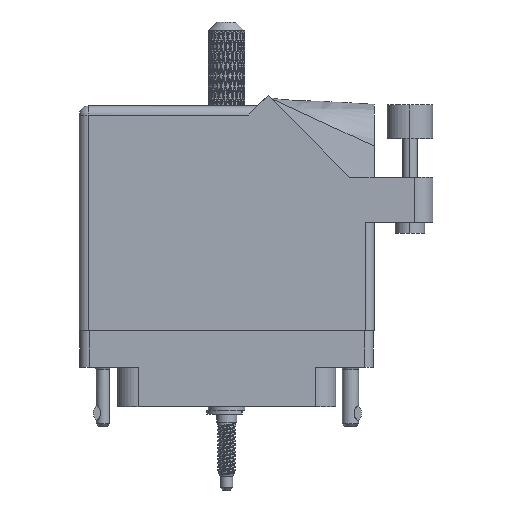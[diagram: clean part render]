
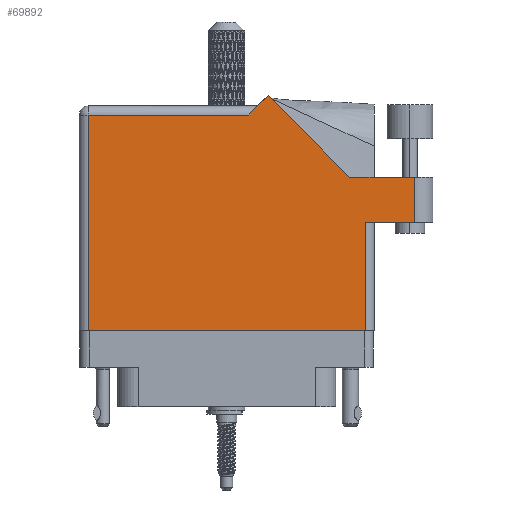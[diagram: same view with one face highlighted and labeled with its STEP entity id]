
A CAD part, front view. The second image highlights one B-rep face of the part: STEP entity #69892.
In plain terms, the highlighted face is planar.
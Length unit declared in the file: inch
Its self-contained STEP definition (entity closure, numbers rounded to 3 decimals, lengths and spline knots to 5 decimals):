
#70 = DIRECTION ( 'NONE',  ( 0., 1., 0. ) ) ;
#1159 = CARTESIAN_POINT ( 'NONE',  ( -0.943, -0.1, 0.455 ) ) ;
#1504 = ORIENTED_EDGE ( 'NONE', *, *, #32686, .T. ) ;
#2131 = EDGE_CURVE ( 'NONE', #22800, #91411, #106348, .T. ) ;
#4507 = DIRECTION ( 'NONE',  ( 1., 0., 0. ) ) ;
#7946 = VECTOR ( 'NONE', #80588, 39.37008 ) ;
#8177 = CARTESIAN_POINT ( 'NONE',  ( 0.83942, 0.944, 0.455 ) ) ;
#8444 = EDGE_LOOP ( 'NONE', ( #69214, #48696, #98636, #86304, #88115, #1504, #74698, #107343, #59697 ) ) ;
#13802 = CARTESIAN_POINT ( 'NONE',  ( 0.28271, 1.50071, 0.455 ) ) ;
#15116 = DIRECTION ( 'NONE',  ( -1., 0., 0. ) ) ;
#17156 = DIRECTION ( 'NONE',  ( -1., 0., 0. ) ) ;
#17251 = VERTEX_POINT ( 'NONE', #101605 ) ;
#18309 = LINE ( 'NONE', #50708, #41927 ) ;
#22800 = VERTEX_POINT ( 'NONE', #23047 ) ;
#23047 = CARTESIAN_POINT ( 'NONE',  ( -0.943, 1.368, 0.455 ) ) ;
#28487 = VERTEX_POINT ( 'NONE', #80352 ) ;
#31535 = LINE ( 'NONE', #88397, #7946 ) ;
#31931 = VECTOR ( 'NONE', #17156, 39.37008 ) ;
#32572 = VECTOR ( 'NONE', #74774, 39.37008 ) ;
#32627 = PLANE ( 'NONE',  #54990 ) ;
#32686 = EDGE_CURVE ( 'NONE', #17251, #22800, #87689, .T. ) ;
#33299 = CARTESIAN_POINT ( 'NONE',  ( 0.943, -0.1, 0.455 ) ) ;
#34032 = LINE ( 'NONE', #81395, #32572 ) ;
#36091 = DIRECTION ( 'NONE',  ( 0., -1., 0. ) ) ;
#36533 = CARTESIAN_POINT ( 'NONE',  ( 0.943, 0.637, 0.455 ) ) ;
#38821 = CARTESIAN_POINT ( 'NONE',  ( 0.212, 1.43, 0.455 ) ) ;
#41927 = VECTOR ( 'NONE', #4507, 39.37008 ) ;
#47375 = EDGE_CURVE ( 'NONE', #63339, #50815, #65815, .T. ) ;
#48696 = ORIENTED_EDGE ( 'NONE', *, *, #92833, .T. ) ;
#49235 = DIRECTION ( 'NONE',  ( -0.707, 0.707, 0. ) ) ;
#49749 = EDGE_CURVE ( 'NONE', #81736, #74906, #18309, .T. ) ;
#50257 = EDGE_CURVE ( 'NONE', #93509, #81736, #82212, .T. ) ;
#50708 = CARTESIAN_POINT ( 'NONE',  ( 1.005, 0.637, 0.455 ) ) ;
#50815 = VERTEX_POINT ( 'NONE', #13802 ) ;
#54990 = AXIS2_PLACEMENT_3D ( 'NONE', #104439, #94807, #15116 ) ;
#55980 = DIRECTION ( 'NONE',  ( -0.707, -0.707, 0. ) ) ;
#56843 = EDGE_CURVE ( 'NONE', #50815, #17251, #106384, .T. ) ;
#59697 = ORIENTED_EDGE ( 'NONE', *, *, #50257, .T. ) ;
#60405 = CARTESIAN_POINT ( 'NONE',  ( -0.943, -0.1, 0.455 ) ) ;
#63339 = VERTEX_POINT ( 'NONE', #8177 ) ;
#63896 = CARTESIAN_POINT ( 'NONE',  ( 0.943, 0.637, 0.455 ) ) ;
#65815 = LINE ( 'NONE', #99767, #76390 ) ;
#67257 = CARTESIAN_POINT ( 'NONE',  ( 1.28, 0.637, 0.455 ) ) ;
#69214 = ORIENTED_EDGE ( 'NONE', *, *, #49749, .T. ) ;
#69701 = VECTOR ( 'NONE', #70, 39.37008 ) ;
#69892 = ADVANCED_FACE ( 'NONE', ( #75536 ), #32627, .F. ) ;
#74459 = VECTOR ( 'NONE', #55980, 39.37008 ) ;
#74698 = ORIENTED_EDGE ( 'NONE', *, *, #2131, .T. ) ;
#74774 = DIRECTION ( 'NONE',  ( 1., 0., 0. ) ) ;
#74906 = VERTEX_POINT ( 'NONE', #67257 ) ;
#75536 = FACE_OUTER_BOUND ( 'NONE', #8444, .T. ) ;
#76390 = VECTOR ( 'NONE', #49235, 39.37008 ) ;
#79797 = EDGE_CURVE ( 'NONE', #91411, #93509, #34032, .T. ) ;
#80352 = CARTESIAN_POINT ( 'NONE',  ( 1.28, 0.944, 0.455 ) ) ;
#80588 = DIRECTION ( 'NONE',  ( 0., 1., 0. ) ) ;
#81395 = CARTESIAN_POINT ( 'NONE',  ( -1.005, -0.1, 0.455 ) ) ;
#81736 = VERTEX_POINT ( 'NONE', #63896 ) ;
#82212 = LINE ( 'NONE', #36533, #69701 ) ;
#82765 = VECTOR ( 'NONE', #36091, 39.37008 ) ;
#86304 = ORIENTED_EDGE ( 'NONE', *, *, #47375, .T. ) ;
#87217 = CARTESIAN_POINT ( 'NONE',  ( 1.405, 0.944, 0.455 ) ) ;
#87689 = LINE ( 'NONE', #105294, #31931 ) ;
#88115 = ORIENTED_EDGE ( 'NONE', *, *, #56843, .T. ) ;
#88397 = CARTESIAN_POINT ( 'NONE',  ( 1.28, 0.944, 0.455 ) ) ;
#91411 = VERTEX_POINT ( 'NONE', #60405 ) ;
#92783 = EDGE_CURVE ( 'NONE', #28487, #63339, #109304, .T. ) ;
#92833 = EDGE_CURVE ( 'NONE', #74906, #28487, #31535, .T. ) ;
#93509 = VERTEX_POINT ( 'NONE', #33299 ) ;
#94807 = DIRECTION ( 'NONE',  ( 0., 0., -1. ) ) ;
#98268 = VECTOR ( 'NONE', #103447, 39.37008 ) ;
#98636 = ORIENTED_EDGE ( 'NONE', *, *, #92783, .T. ) ;
#99767 = CARTESIAN_POINT ( 'NONE',  ( 0.83942, 0.944, 0.455 ) ) ;
#101605 = CARTESIAN_POINT ( 'NONE',  ( 0.15, 1.368, 0.455 ) ) ;
#103447 = DIRECTION ( 'NONE',  ( -1., 0., 0. ) ) ;
#104439 = CARTESIAN_POINT ( 'NONE',  ( -1.005, 1.43, 0.455 ) ) ;
#105294 = CARTESIAN_POINT ( 'NONE',  ( -1.005, 1.368, 0.455 ) ) ;
#106348 = LINE ( 'NONE', #1159, #82765 ) ;
#106384 = LINE ( 'NONE', #38821, #74459 ) ;
#107343 = ORIENTED_EDGE ( 'NONE', *, *, #79797, .T. ) ;
#109304 = LINE ( 'NONE', #87217, #98268 ) ;
